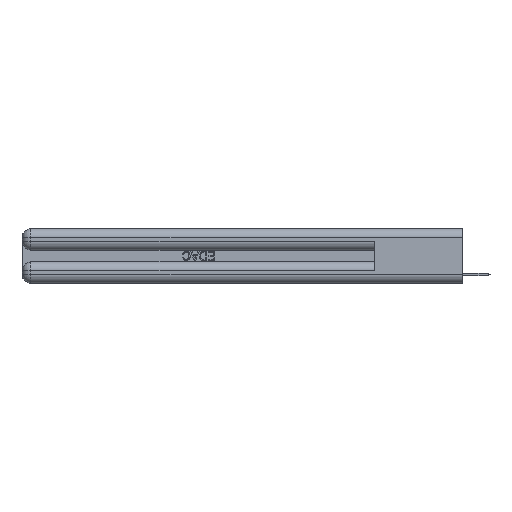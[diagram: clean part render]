
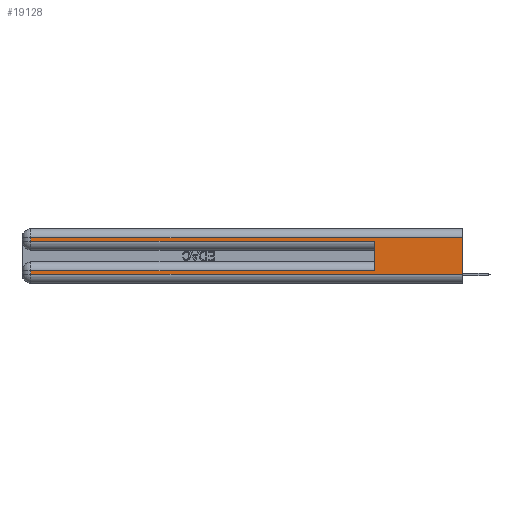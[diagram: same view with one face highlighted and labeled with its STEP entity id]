
A CAD part, left-side view. The second image highlights one B-rep face of the part: STEP entity #19128.
In plain terms, the highlighted planar face has unit normal (-1, 0, 0).
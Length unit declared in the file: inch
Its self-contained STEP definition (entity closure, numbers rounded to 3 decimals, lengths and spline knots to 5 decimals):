
#1171 = CARTESIAN_POINT ( 'NONE',  ( 0., 2.94, 0.285 ) ) ;
#1345 = DIRECTION ( 'NONE',  ( 0., 0., -1. ) ) ;
#1556 = CARTESIAN_POINT ( 'NONE',  ( 0., 2.94, 0.37 ) ) ;
#1692 = ORIENTED_EDGE ( 'NONE', *, *, #24639, .T. ) ;
#2793 = CARTESIAN_POINT ( 'NONE',  ( 0., 0., 0.31 ) ) ;
#3190 = LINE ( 'NONE', #28070, #18558 ) ;
#3457 = FACE_OUTER_BOUND ( 'NONE', #12083, .T. ) ;
#3667 = VECTOR ( 'NONE', #15444, 39.37008 ) ;
#4061 = VERTEX_POINT ( 'NONE', #1171 ) ;
#4233 = VERTEX_POINT ( 'NONE', #17829 ) ;
#4655 = VECTOR ( 'NONE', #28894, 39.37008 ) ;
#5002 = CARTESIAN_POINT ( 'NONE',  ( 0., 0.6, 0.285 ) ) ;
#5199 = VECTOR ( 'NONE', #1345, 39.37008 ) ;
#5718 = DIRECTION ( 'NONE',  ( 0., 0., -1. ) ) ;
#5761 = AXIS2_PLACEMENT_3D ( 'NONE', #24279, #10880, #22216 ) ;
#5823 = ORIENTED_EDGE ( 'NONE', *, *, #11323, .T. ) ;
#6598 = LINE ( 'NONE', #1556, #5199 ) ;
#7948 = CARTESIAN_POINT ( 'NONE',  ( 0., 0., 0.37 ) ) ;
#8603 = ORIENTED_EDGE ( 'NONE', *, *, #11221, .F. ) ;
#8625 = PLANE ( 'NONE',  #5761 ) ;
#9057 = VECTOR ( 'NONE', #11687, 39.37008 ) ;
#9728 = VERTEX_POINT ( 'NONE', #13819 ) ;
#10001 = DIRECTION ( 'NONE',  ( 0., 0., -1. ) ) ;
#10288 = EDGE_CURVE ( 'NONE', #17005, #27894, #10812, .T. ) ;
#10812 = LINE ( 'NONE', #7948, #22000 ) ;
#10880 = DIRECTION ( 'NONE',  ( 1., 0., 0. ) ) ;
#11221 = EDGE_CURVE ( 'NONE', #13320, #17014, #20932, .T. ) ;
#11323 = EDGE_CURVE ( 'NONE', #23861, #4233, #6598, .T. ) ;
#11623 = CARTESIAN_POINT ( 'NONE',  ( 0., 0., 0.31 ) ) ;
#11687 = DIRECTION ( 'NONE',  ( 0., 0., 1. ) ) ;
#11691 = LINE ( 'NONE', #28811, #3667 ) ;
#12083 = EDGE_LOOP ( 'NONE', ( #23507, #14285, #1692, #28079, #8603, #23821, #5823, #24109 ) ) ;
#12494 = EDGE_CURVE ( 'NONE', #17005, #9728, #16349, .T. ) ;
#13320 = VERTEX_POINT ( 'NONE', #23890 ) ;
#13819 = CARTESIAN_POINT ( 'NONE',  ( 0., 2.94, 0.31 ) ) ;
#14285 = ORIENTED_EDGE ( 'NONE', *, *, #12494, .T. ) ;
#15175 = CARTESIAN_POINT ( 'NONE',  ( 0., 0., 0.06 ) ) ;
#15444 = DIRECTION ( 'NONE',  ( 0., -1., 0. ) ) ;
#15643 = VECTOR ( 'NONE', #18941, 39.37008 ) ;
#16349 = LINE ( 'NONE', #11623, #15643 ) ;
#16357 = EDGE_CURVE ( 'NONE', #4233, #27894, #27033, .T. ) ;
#17005 = VERTEX_POINT ( 'NONE', #2793 ) ;
#17014 = VERTEX_POINT ( 'NONE', #5002 ) ;
#17022 = VECTOR ( 'NONE', #10001, 39.37008 ) ;
#17311 = EDGE_CURVE ( 'NONE', #13320, #23861, #3190, .T. ) ;
#17829 = CARTESIAN_POINT ( 'NONE',  ( 0., 2.94, 0.06 ) ) ;
#18558 = VECTOR ( 'NONE', #23572, 39.37008 ) ;
#18637 = CARTESIAN_POINT ( 'NONE',  ( 0., 0.6, 0.145 ) ) ;
#18794 = CARTESIAN_POINT ( 'NONE',  ( 0., 2.94, 0.37 ) ) ;
#18941 = DIRECTION ( 'NONE',  ( 0., 1., 0. ) ) ;
#19128 = ADVANCED_FACE ( 'NONE', ( #3457 ), #8625, .F. ) ;
#20932 = LINE ( 'NONE', #18637, #9057 ) ;
#22000 = VECTOR ( 'NONE', #5718, 39.37008 ) ;
#22211 = LINE ( 'NONE', #18794, #17022 ) ;
#22216 = DIRECTION ( 'NONE',  ( 0., 0., -1. ) ) ;
#23507 = ORIENTED_EDGE ( 'NONE', *, *, #10288, .F. ) ;
#23572 = DIRECTION ( 'NONE',  ( 0., 1., 0. ) ) ;
#23821 = ORIENTED_EDGE ( 'NONE', *, *, #17311, .T. ) ;
#23861 = VERTEX_POINT ( 'NONE', #28553 ) ;
#23890 = CARTESIAN_POINT ( 'NONE',  ( 0., 0.6, 0.085 ) ) ;
#24109 = ORIENTED_EDGE ( 'NONE', *, *, #16357, .T. ) ;
#24279 = CARTESIAN_POINT ( 'NONE',  ( 0., 0., 0.37 ) ) ;
#24639 = EDGE_CURVE ( 'NONE', #9728, #4061, #22211, .T. ) ;
#25574 = EDGE_CURVE ( 'NONE', #4061, #17014, #11691, .T. ) ;
#26562 = CARTESIAN_POINT ( 'NONE',  ( 0., 0., 0.06 ) ) ;
#27033 = LINE ( 'NONE', #26562, #4655 ) ;
#27894 = VERTEX_POINT ( 'NONE', #15175 ) ;
#28070 = CARTESIAN_POINT ( 'NONE',  ( 0., 0., 0.085 ) ) ;
#28079 = ORIENTED_EDGE ( 'NONE', *, *, #25574, .T. ) ;
#28553 = CARTESIAN_POINT ( 'NONE',  ( 0., 2.94, 0.085 ) ) ;
#28811 = CARTESIAN_POINT ( 'NONE',  ( 0., 0., 0.285 ) ) ;
#28894 = DIRECTION ( 'NONE',  ( 0., -1., 0. ) ) ;
